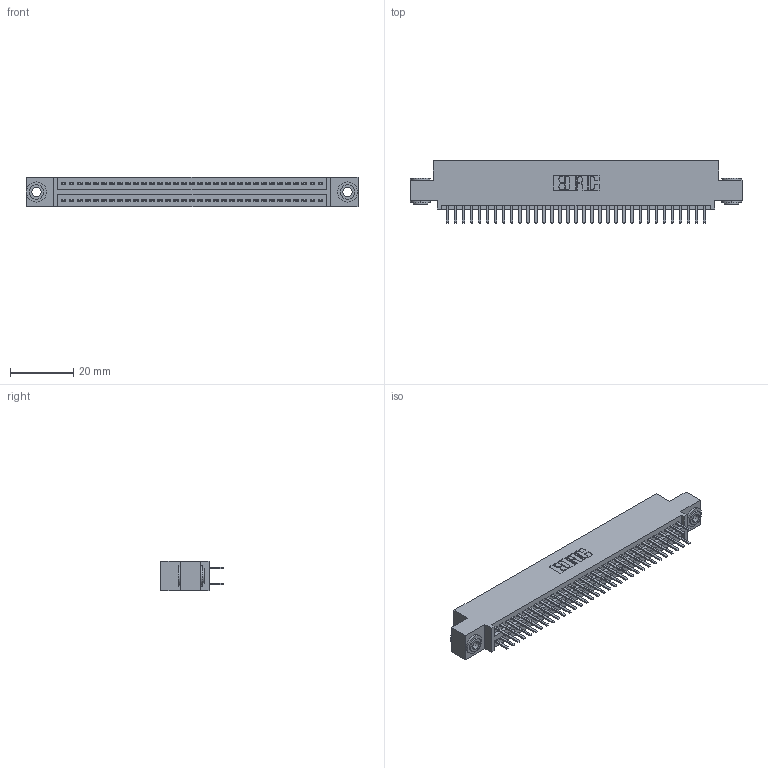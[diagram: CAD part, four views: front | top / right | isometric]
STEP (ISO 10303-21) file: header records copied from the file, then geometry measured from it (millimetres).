
FILE_DESCRIPTION (( 'STEP AP203' ), '1' );
FILE_NAME ('395-066-520-503.STEP', '2018-11-25T00:44:53', ( '' ), ( '' ), 'SwSTEP 2.0', 'SolidWorks 2016', '' );
FILE_SCHEMA (( 'CONFIG_CONTROL_DESIGN' ));
Length unit declared in the file: inch
Products named in the file (4): 395-066-520-503; 345 Part_0.110 Offset - 0.156 Dia-TH; 345-250-002_345-250-002-102; 345-292-001_345-293-120
Assembly tree (69 placements, depth 2):
  395-066-520-503
    345 Part_0.110 Offset - 0.156 Dia-TH
    345-292-001_345-293-120  x66
    345-250-002_345-250-002-102  x2
Bounding box: 105.03 x 19.68 x 9.4 mm (x, y, z)
Volume: 10036.1 mm3; surface area: 14896.7 mm2
Topology: 69 solids, 69 shells, 3732 faces, 10791 edges, 7014 vertices
Faces by surface type: plane 2404, cylinder 1320, cone 8
Entity records: 28000 total; most frequent: CARTESIAN_POINT 4691, ORIENTED_EDGE 4606, DIRECTION 4165, EDGE_CURVE 2303, VECTOR 2011, LINE 2011, VERTEX_POINT 1530, AXIS2_PLACEMENT_3D 1077
